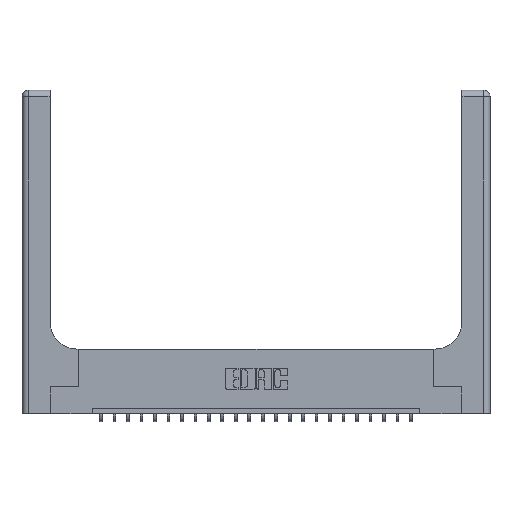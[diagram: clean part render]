
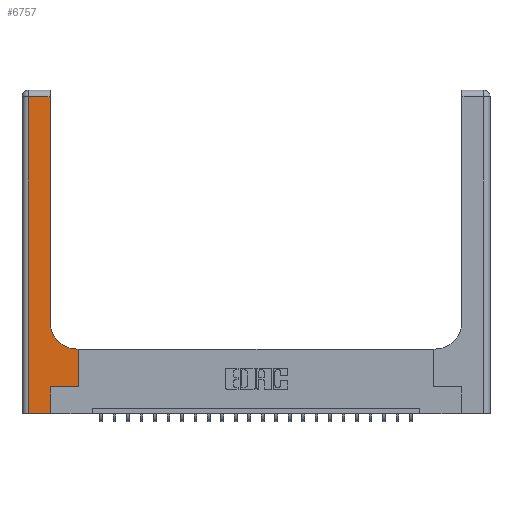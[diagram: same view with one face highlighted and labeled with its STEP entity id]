
A CAD part, top view. The second image highlights one B-rep face of the part: STEP entity #6757.
In plain terms, the highlighted planar face has unit normal (0, 0, 1).
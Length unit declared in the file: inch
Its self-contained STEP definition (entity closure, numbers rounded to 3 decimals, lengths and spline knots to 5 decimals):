
#72 = CARTESIAN_POINT ( 'NONE',  ( 0.528, 0.6, 0.37 ) ) ;
#464 = EDGE_CURVE ( 'NONE', #12660, #3891, #10490, .T. ) ;
#1203 = LINE ( 'NONE', #20762, #16715 ) ;
#1334 = CARTESIAN_POINT ( 'NONE',  ( 0.265, 0., 0.37 ) ) ;
#1605 = ORIENTED_EDGE ( 'NONE', *, *, #16131, .T. ) ;
#1757 = ORIENTED_EDGE ( 'NONE', *, *, #464, .T. ) ;
#2462 = DIRECTION ( 'NONE',  ( 0., 0., -1. ) ) ;
#2549 = VECTOR ( 'NONE', #3107, 39.37008 ) ;
#2642 = LINE ( 'NONE', #18927, #20932 ) ;
#3107 = DIRECTION ( 'NONE',  ( -1., 0., 0. ) ) ;
#3741 = DIRECTION ( 'NONE',  ( 1., 0., 0. ) ) ;
#3891 = VERTEX_POINT ( 'NONE', #1334 ) ;
#4439 = ORIENTED_EDGE ( 'NONE', *, *, #15245, .T. ) ;
#4591 = CARTESIAN_POINT ( 'NONE',  ( 0., 3., 0.37 ) ) ;
#4734 = VERTEX_POINT ( 'NONE', #13125 ) ;
#4822 = DIRECTION ( 'NONE',  ( 1., 0., 0. ) ) ;
#4957 = LINE ( 'NONE', #12035, #9300 ) ;
#5303 = LINE ( 'NONE', #5658, #16928 ) ;
#5658 = CARTESIAN_POINT ( 'NONE',  ( 0.265, 0., 0.37 ) ) ;
#6485 = DIRECTION ( 'NONE',  ( 0., 1., 0. ) ) ;
#6562 = LINE ( 'NONE', #15286, #14634 ) ;
#6717 = EDGE_CURVE ( 'NONE', #20333, #12660, #6562, .T. ) ;
#6757 = ADVANCED_FACE ( 'NONE', ( #22177 ), #22400, .F. ) ;
#6884 = CARTESIAN_POINT ( 'NONE',  ( 0., 0., 0.37 ) ) ;
#8036 = DIRECTION ( 'NONE',  ( -1., 0., 0. ) ) ;
#8702 = EDGE_CURVE ( 'NONE', #4734, #16350, #21431, .T. ) ;
#8704 = ORIENTED_EDGE ( 'NONE', *, *, #10885, .T. ) ;
#9300 = VECTOR ( 'NONE', #22420, 39.37008 ) ;
#9596 = CARTESIAN_POINT ( 'NONE',  ( 0.528, 0.25, 0.37 ) ) ;
#9704 = ORIENTED_EDGE ( 'NONE', *, *, #22555, .T. ) ;
#9705 = DIRECTION ( 'NONE',  ( -1., 0., 0. ) ) ;
#9774 = EDGE_CURVE ( 'NONE', #17527, #17699, #1203, .T. ) ;
#10007 = VERTEX_POINT ( 'NONE', #11640 ) ;
#10115 = CARTESIAN_POINT ( 'NONE',  ( 0., 2.94, 0.37 ) ) ;
#10490 = LINE ( 'NONE', #6884, #22760 ) ;
#10755 = CARTESIAN_POINT ( 'NONE',  ( 0.265, 0.25, 0.37 ) ) ;
#10885 = EDGE_CURVE ( 'NONE', #16350, #10007, #2642, .T. ) ;
#10957 = VERTEX_POINT ( 'NONE', #72 ) ;
#11443 = CARTESIAN_POINT ( 'NONE',  ( 0.26, 0.85, 0.37 ) ) ;
#11558 = ORIENTED_EDGE ( 'NONE', *, *, #9774, .T. ) ;
#11559 = DIRECTION ( 'NONE',  ( 0., -1., 0. ) ) ;
#11640 = CARTESIAN_POINT ( 'NONE',  ( 0.26, 2.94, 0.37 ) ) ;
#12035 = CARTESIAN_POINT ( 'NONE',  ( 0.528, 0.25, 0.37 ) ) ;
#12086 = LINE ( 'NONE', #10115, #15809 ) ;
#12660 = VERTEX_POINT ( 'NONE', #15613 ) ;
#13109 = EDGE_LOOP ( 'NONE', ( #8704, #4439, #15925, #1757, #1605, #11558, #9704, #14567, #22079 ) ) ;
#13125 = CARTESIAN_POINT ( 'NONE',  ( 0.51, 0.6, 0.37 ) ) ;
#14355 = AXIS2_PLACEMENT_3D ( 'NONE', #18412, #2462, #18078 ) ;
#14567 = ORIENTED_EDGE ( 'NONE', *, *, #20978, .T. ) ;
#14590 = DIRECTION ( 'NONE',  ( 0., 1., 0. ) ) ;
#14634 = VECTOR ( 'NONE', #11559, 39.37008 ) ;
#15245 = EDGE_CURVE ( 'NONE', #10007, #20333, #12086, .T. ) ;
#15286 = CARTESIAN_POINT ( 'NONE',  ( 0.06, 3., 0.37 ) ) ;
#15443 = CARTESIAN_POINT ( 'NONE',  ( 0.26, 0.6, 0.37 ) ) ;
#15613 = CARTESIAN_POINT ( 'NONE',  ( 0.06, 0., 0.37 ) ) ;
#15789 = LINE ( 'NONE', #15443, #2549 ) ;
#15809 = VECTOR ( 'NONE', #8036, 39.37008 ) ;
#15925 = ORIENTED_EDGE ( 'NONE', *, *, #6717, .T. ) ;
#16131 = EDGE_CURVE ( 'NONE', #3891, #17527, #5303, .T. ) ;
#16350 = VERTEX_POINT ( 'NONE', #11443 ) ;
#16538 = CARTESIAN_POINT ( 'NONE',  ( 0.06, 2.94, 0.37 ) ) ;
#16715 = VECTOR ( 'NONE', #4822, 39.37008 ) ;
#16928 = VECTOR ( 'NONE', #14590, 39.37008 ) ;
#17527 = VERTEX_POINT ( 'NONE', #10755 ) ;
#17699 = VERTEX_POINT ( 'NONE', #9596 ) ;
#18004 = AXIS2_PLACEMENT_3D ( 'NONE', #4591, #20645, #9705 ) ;
#18078 = DIRECTION ( 'NONE',  ( 1., 0., 0. ) ) ;
#18412 = CARTESIAN_POINT ( 'NONE',  ( 0.51, 0.85, 0.37 ) ) ;
#18927 = CARTESIAN_POINT ( 'NONE',  ( 0.26, 3., 0.37 ) ) ;
#20333 = VERTEX_POINT ( 'NONE', #16538 ) ;
#20645 = DIRECTION ( 'NONE',  ( 0., 0., -1. ) ) ;
#20762 = CARTESIAN_POINT ( 'NONE',  ( 0.265, 0.25, 0.37 ) ) ;
#20932 = VECTOR ( 'NONE', #6485, 39.37008 ) ;
#20978 = EDGE_CURVE ( 'NONE', #10957, #4734, #15789, .T. ) ;
#21431 = CIRCLE ( 'NONE', #14355, 0.25 ) ;
#22079 = ORIENTED_EDGE ( 'NONE', *, *, #8702, .T. ) ;
#22177 = FACE_OUTER_BOUND ( 'NONE', #13109, .T. ) ;
#22400 = PLANE ( 'NONE',  #18004 ) ;
#22420 = DIRECTION ( 'NONE',  ( 0., 1., 0. ) ) ;
#22555 = EDGE_CURVE ( 'NONE', #17699, #10957, #4957, .T. ) ;
#22760 = VECTOR ( 'NONE', #3741, 39.37008 ) ;
